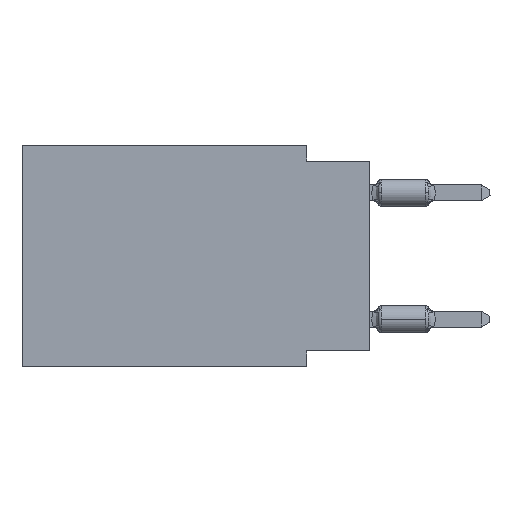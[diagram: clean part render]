
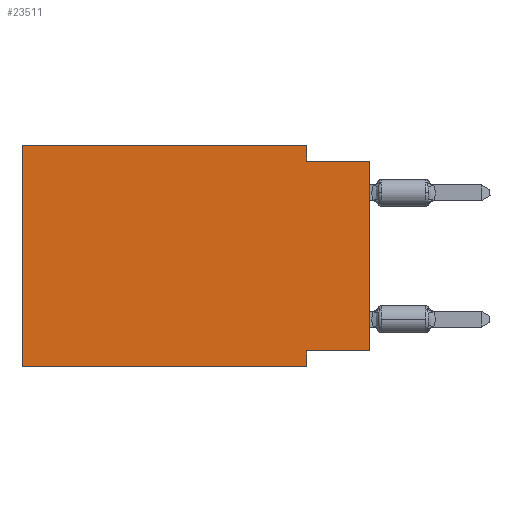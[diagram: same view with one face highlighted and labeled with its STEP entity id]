
A CAD part, left-side view. The second image highlights one B-rep face of the part: STEP entity #23511.
In plain terms, the highlighted planar face has unit normal (-1, 0, 0).
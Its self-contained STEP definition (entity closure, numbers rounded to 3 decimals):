
#394 = LINE ( 'NONE', #16204, #22289 ) ;
#757 = CARTESIAN_POINT ( 'NONE',  ( 0., 13.97, -8.89 ) ) ;
#926 = LINE ( 'NONE', #18922, #11874 ) ;
#1122 = AXIS2_PLACEMENT_3D ( 'NONE', #21408, #25935, #15262 ) ;
#1246 = CARTESIAN_POINT ( 'NONE',  ( 0., 13.97, 0. ) ) ;
#1720 = ORIENTED_EDGE ( 'NONE', *, *, #26086, .T. ) ;
#1831 = LINE ( 'NONE', #21722, #15230 ) ;
#2071 = LINE ( 'NONE', #10860, #26836 ) ;
#2729 = VECTOR ( 'NONE', #5104, 1000. ) ;
#2932 = ORIENTED_EDGE ( 'NONE', *, *, #4709, .F. ) ;
#3050 = DIRECTION ( 'NONE',  ( 0., -1., 0. ) ) ;
#3567 = FACE_OUTER_BOUND ( 'NONE', #5889, .T. ) ;
#3674 = VERTEX_POINT ( 'NONE', #19144 ) ;
#4709 = EDGE_CURVE ( 'NONE', #3674, #18546, #23896, .T. ) ;
#5104 = DIRECTION ( 'NONE',  ( 0., 0., 1. ) ) ;
#5622 = DIRECTION ( 'NONE',  ( 0., 0., -1. ) ) ;
#5805 = CARTESIAN_POINT ( 'NONE',  ( 0., 2.54, -0.635 ) ) ;
#5889 = EDGE_LOOP ( 'NONE', ( #1720, #14521, #21790, #2932, #21849, #6032, #14562, #12351 ) ) ;
#6032 = ORIENTED_EDGE ( 'NONE', *, *, #19796, .T. ) ;
#6145 = CARTESIAN_POINT ( 'NONE',  ( 0., 0., -0.635 ) ) ;
#6524 = VECTOR ( 'NONE', #15013, 1000. ) ;
#7150 = CARTESIAN_POINT ( 'NONE',  ( 0., 13.97, -8.89 ) ) ;
#9022 = CARTESIAN_POINT ( 'NONE',  ( 0., 0., -8.255 ) ) ;
#9121 = EDGE_CURVE ( 'NONE', #18546, #14345, #926, .T. ) ;
#10860 = CARTESIAN_POINT ( 'NONE',  ( 0., 13.97, 0. ) ) ;
#10996 = DIRECTION ( 'NONE',  ( 0., 0., 1. ) ) ;
#11874 = VECTOR ( 'NONE', #5622, 1000. ) ;
#11974 = CARTESIAN_POINT ( 'NONE',  ( 0., 0., 0. ) ) ;
#12044 = EDGE_CURVE ( 'NONE', #19108, #3674, #2071, .T. ) ;
#12351 = ORIENTED_EDGE ( 'NONE', *, *, #14446, .F. ) ;
#12820 = LINE ( 'NONE', #23626, #28371 ) ;
#13629 = CARTESIAN_POINT ( 'NONE',  ( 0., 2.54, -8.255 ) ) ;
#14345 = VERTEX_POINT ( 'NONE', #5805 ) ;
#14446 = EDGE_CURVE ( 'NONE', #28409, #16196, #1831, .T. ) ;
#14521 = ORIENTED_EDGE ( 'NONE', *, *, #17923, .F. ) ;
#14562 = ORIENTED_EDGE ( 'NONE', *, *, #18029, .F. ) ;
#14874 = VECTOR ( 'NONE', #16270, 1000. ) ;
#14890 = CARTESIAN_POINT ( 'NONE',  ( 0., 2.54, -8.89 ) ) ;
#15013 = DIRECTION ( 'NONE',  ( 0., -1., 0. ) ) ;
#15230 = VECTOR ( 'NONE', #28728, 1000. ) ;
#15262 = DIRECTION ( 'NONE',  ( 0., 0., -1. ) ) ;
#16196 = VERTEX_POINT ( 'NONE', #13629 ) ;
#16204 = CARTESIAN_POINT ( 'NONE',  ( 0., 0., -0.635 ) ) ;
#16270 = DIRECTION ( 'NONE',  ( 0., -1., 0. ) ) ;
#17315 = PLANE ( 'NONE',  #1122 ) ;
#17923 = EDGE_CURVE ( 'NONE', #14345, #25757, #394, .T. ) ;
#18029 = EDGE_CURVE ( 'NONE', #16196, #28376, #12820, .T. ) ;
#18466 = LINE ( 'NONE', #757, #14874 ) ;
#18546 = VERTEX_POINT ( 'NONE', #19370 ) ;
#18922 = CARTESIAN_POINT ( 'NONE',  ( 0., 2.54, 0. ) ) ;
#19108 = VERTEX_POINT ( 'NONE', #7150 ) ;
#19125 = DIRECTION ( 'NONE',  ( 0., 0., -1. ) ) ;
#19144 = CARTESIAN_POINT ( 'NONE',  ( 0., 13.97, 0. ) ) ;
#19370 = CARTESIAN_POINT ( 'NONE',  ( 0., 2.54, 0. ) ) ;
#19796 = EDGE_CURVE ( 'NONE', #19108, #28376, #18466, .T. ) ;
#21408 = CARTESIAN_POINT ( 'NONE',  ( 0., 13.97, 0. ) ) ;
#21722 = CARTESIAN_POINT ( 'NONE',  ( 0., 0., -8.255 ) ) ;
#21790 = ORIENTED_EDGE ( 'NONE', *, *, #9121, .F. ) ;
#21849 = ORIENTED_EDGE ( 'NONE', *, *, #12044, .F. ) ;
#22289 = VECTOR ( 'NONE', #3050, 1000. ) ;
#23052 = LINE ( 'NONE', #11974, #2729 ) ;
#23511 = ADVANCED_FACE ( 'NONE', ( #3567 ), #17315, .F. ) ;
#23626 = CARTESIAN_POINT ( 'NONE',  ( 0., 2.54, -8.89 ) ) ;
#23896 = LINE ( 'NONE', #1246, #6524 ) ;
#25757 = VERTEX_POINT ( 'NONE', #6145 ) ;
#25935 = DIRECTION ( 'NONE',  ( 1., 0., 0. ) ) ;
#26086 = EDGE_CURVE ( 'NONE', #28409, #25757, #23052, .T. ) ;
#26836 = VECTOR ( 'NONE', #10996, 1000. ) ;
#28371 = VECTOR ( 'NONE', #19125, 1000. ) ;
#28376 = VERTEX_POINT ( 'NONE', #14890 ) ;
#28409 = VERTEX_POINT ( 'NONE', #9022 ) ;
#28728 = DIRECTION ( 'NONE',  ( 0., 1., 0. ) ) ;
